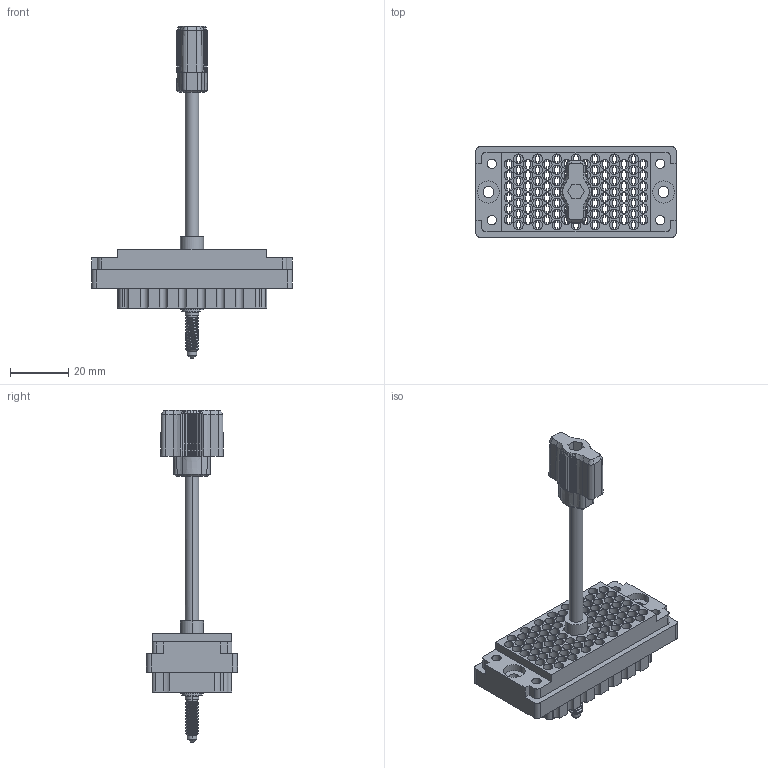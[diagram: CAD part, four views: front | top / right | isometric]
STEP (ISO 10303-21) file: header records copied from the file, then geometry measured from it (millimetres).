
FILE_DESCRIPTION (( 'STEP AP203' ), '1' );
FILE_NAME ('516-090-000-205.STEP', '2020-03-06T16:05:13', ( '' ), ( '' ), 'SwSTEP 2.0', 'SolidWorks 2016', '' );
FILE_SCHEMA (( 'CONFIG_CONTROL_DESIGN' ));
Length unit declared in the file: inch
Products named in the file (9): 516-253-190-107; 516-251-095-100; Grub Screw; 516-254-091-109; 516-090-000-205; 516-250-091-111; 516-253-095-100; Actuating Screw Assy 090-120; 516 Part Receptacle_090
Assembly tree (9 placements, depth 3):
  516-090-000-205
    516 Part Receptacle_090
    Actuating Screw Assy 090-120
      516-251-095-100
      516-254-091-109
      516-253-095-100  x2
      516-253-190-107
      516-250-091-111
      Grub Screw
Bounding box: 69.04 x 31.34 x 114.34 mm (x, y, z)
Volume: 24771.3 mm3; surface area: 33799.2 mm2
Topology: 8 solids, 8 shells, 2227 faces, 6477 edges, 4290 vertices
Faces by surface type: plane 1487, cylinder 661, cone 62, bspline 17
Entity records: 81490 total; most frequent: CARTESIAN_POINT 20269, ORIENTED_EDGE 12930, DIRECTION 12379, EDGE_CURVE 6465, LINE 4591, VECTOR 4591, VERTEX_POINT 4282, AXIS2_PLACEMENT_3D 3894
